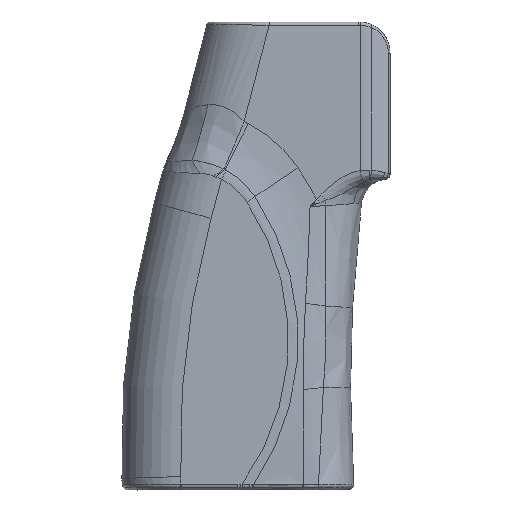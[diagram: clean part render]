
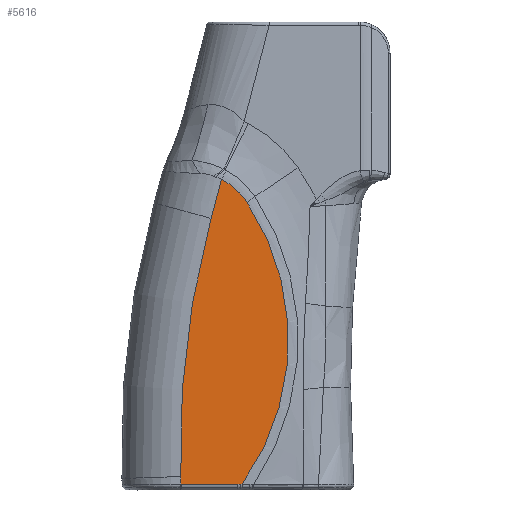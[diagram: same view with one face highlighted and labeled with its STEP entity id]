
A CAD part, left-side view. The second image highlights one B-rep face of the part: STEP entity #5616.
In plain terms, the highlighted planar face has unit normal (-1, 0, 0).
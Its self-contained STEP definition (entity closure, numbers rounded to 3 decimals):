
#102=PLANE('',#6028);
#186=LINE('',#9908,#366);
#366=VECTOR('',#6651,10.);
#677=FACE_OUTER_BOUND('',#1051,.T.);
#1051=EDGE_LOOP('',(#4062,#4063,#4064,#4065,#4066,#4067,#4068,#4069,#4070,
#4071));
#1429=CIRCLE('',#6029,50.737);
#1430=CIRCLE('',#6030,13.96);
#1431=CIRCLE('',#6031,1010.767);
#1432=CIRCLE('',#6032,178.004);
#1433=CIRCLE('',#6033,103.75);
#1751=B_SPLINE_CURVE_WITH_KNOTS('',3,(#9899,#9900,#9901,#9902),
 .UNSPECIFIED.,.F.,.F.,(4,4),(0.,0.054),.UNSPECIFIED.);
#1753=B_SPLINE_CURVE_WITH_KNOTS('',3,(#9932,#9933,#9934,#9935),
 .UNSPECIFIED.,.F.,.F.,(4,4),(0.,0.001),.UNSPECIFIED.);
#1755=B_SPLINE_CURVE_WITH_KNOTS('',3,(#9956,#9957,#9958,#9959),
 .UNSPECIFIED.,.F.,.F.,(4,4),(0.,0.033),
 .UNSPECIFIED.);
#1761=B_SPLINE_CURVE_WITH_KNOTS('',3,(#10067,#10068,#10069,#10070),
 .UNSPECIFIED.,.F.,.F.,(4,4),(0.,0.001),
 .UNSPECIFIED.);
#2205=VERTEX_POINT('',#9838);
#2207=VERTEX_POINT('',#9889);
#2210=VERTEX_POINT('',#9897);
#2211=VERTEX_POINT('',#9904);
#2213=VERTEX_POINT('',#9925);
#2218=VERTEX_POINT('',#9994);
#2275=VERTEX_POINT('',#10916);
#2276=VERTEX_POINT('',#10918);
#2277=VERTEX_POINT('',#10920);
#2278=VERTEX_POINT('',#10922);
#2842=EDGE_CURVE('',#2210,#2207,#1751,.T.);
#2845=EDGE_CURVE('',#2207,#2211,#186,.T.);
#2848=EDGE_CURVE('',#2211,#2213,#1753,.T.);
#2850=EDGE_CURVE('',#2205,#2210,#1755,.T.);
#2862=EDGE_CURVE('',#2213,#2218,#1761,.T.);
#2949=EDGE_CURVE('',#2275,#2205,#1429,.T.);
#2950=EDGE_CURVE('',#2276,#2275,#1430,.T.);
#2951=EDGE_CURVE('',#2277,#2276,#1431,.T.);
#2952=EDGE_CURVE('',#2278,#2277,#1432,.T.);
#2953=EDGE_CURVE('',#2218,#2278,#1433,.T.);
#4062=ORIENTED_EDGE('',*,*,#2862,.F.);
#4063=ORIENTED_EDGE('',*,*,#2848,.F.);
#4064=ORIENTED_EDGE('',*,*,#2845,.F.);
#4065=ORIENTED_EDGE('',*,*,#2842,.F.);
#4066=ORIENTED_EDGE('',*,*,#2850,.F.);
#4067=ORIENTED_EDGE('',*,*,#2949,.F.);
#4068=ORIENTED_EDGE('',*,*,#2950,.F.);
#4069=ORIENTED_EDGE('',*,*,#2951,.F.);
#4070=ORIENTED_EDGE('',*,*,#2952,.F.);
#4071=ORIENTED_EDGE('',*,*,#2953,.F.);
#5616=ADVANCED_FACE('',(#677),#102,.T.);
#6028=AXIS2_PLACEMENT_3D('',#10915,#6732,#6733);
#6029=AXIS2_PLACEMENT_3D('',#10917,#6734,#6735);
#6030=AXIS2_PLACEMENT_3D('',#10919,#6736,#6737);
#6031=AXIS2_PLACEMENT_3D('',#10921,#6738,#6739);
#6032=AXIS2_PLACEMENT_3D('',#10923,#6740,#6741);
#6033=AXIS2_PLACEMENT_3D('',#10924,#6742,#6743);
#6651=DIRECTION('',(0.,1.,0.));
#6732=DIRECTION('center_axis',(-1.,0.,0.));
#6733=DIRECTION('ref_axis',(0.,-1.,0.));
#6734=DIRECTION('center_axis',(1.,0.,0.));
#6735=DIRECTION('ref_axis',(0.,-0.988,-0.153));
#6736=DIRECTION('center_axis',(1.,0.,0.));
#6737=DIRECTION('ref_axis',(0.,-0.663,0.748));
#6738=DIRECTION('center_axis',(-1.,0.,0.));
#6739=DIRECTION('ref_axis',(0.,-0.966,-0.259));
#6740=DIRECTION('center_axis',(1.,0.,0.));
#6741=DIRECTION('ref_axis',(0.,0.993,0.116));
#6742=DIRECTION('center_axis',(-1.,0.,0.));
#6743=DIRECTION('ref_axis',(0.,-0.999,-0.051));
#9838=CARTESIAN_POINT('',(11.668,-119.652,-65.824));
#9889=CARTESIAN_POINT('',(11.668,-118.787,-65.836));
#9897=CARTESIAN_POINT('',(11.668,-119.325,-65.832));
#9899=CARTESIAN_POINT('Ctrl Pts',(11.668,-119.325,-65.832));
#9900=CARTESIAN_POINT('Ctrl Pts',(11.668,-119.146,-65.835));
#9901=CARTESIAN_POINT('Ctrl Pts',(11.668,-118.967,-65.836));
#9902=CARTESIAN_POINT('Ctrl Pts',(11.668,-118.787,-65.836));
#9904=CARTESIAN_POINT('',(11.668,-107.204,-65.836));
#9908=CARTESIAN_POINT('',(11.668,-119.773,-65.836));
#9925=CARTESIAN_POINT('',(11.668,-107.197,-65.836));
#9932=CARTESIAN_POINT('Ctrl Pts',(11.668,-107.204,-65.836));
#9933=CARTESIAN_POINT('Ctrl Pts',(11.668,-107.202,-65.836));
#9934=CARTESIAN_POINT('Ctrl Pts',(11.668,-107.199,-65.836));
#9935=CARTESIAN_POINT('Ctrl Pts',(11.668,-107.197,-65.836));
#9956=CARTESIAN_POINT('Ctrl Pts',(11.668,-119.652,-65.824));
#9957=CARTESIAN_POINT('Ctrl Pts',(11.668,-119.543,-65.828));
#9958=CARTESIAN_POINT('Ctrl Pts',(11.668,-119.434,-65.831));
#9959=CARTESIAN_POINT('Ctrl Pts',(11.668,-119.325,-65.832));
#9994=CARTESIAN_POINT('',(11.668,-107.19,-65.836));
#10067=CARTESIAN_POINT('Ctrl Pts',(11.668,-107.197,-65.836));
#10068=CARTESIAN_POINT('Ctrl Pts',(11.668,-107.195,-65.836));
#10069=CARTESIAN_POINT('Ctrl Pts',(11.668,-107.193,-65.836));
#10070=CARTESIAN_POINT('Ctrl Pts',(11.668,-107.19,-65.836));
#10915=CARTESIAN_POINT('Origin',(11.668,-118.964,-29.797));
#10916=CARTESIAN_POINT('',(11.668,-120.61,-8.274));
#10917=CARTESIAN_POINT('Origin',(11.668,-78.351,-36.354));
#10918=CARTESIAN_POINT('',(11.668,-115.458,-3.633));
#10919=CARTESIAN_POINT('Origin',(11.668,-108.983,-16.));
#10920=CARTESIAN_POINT('',(11.668,-113.317,-11.621));
#10921=CARTESIAN_POINT('Origin',(11.668,861.892,254.118));
#10922=CARTESIAN_POINT('',(11.668,-107.15,-64.253));
#10923=CARTESIAN_POINT('Origin',(11.668,-285.059,-58.42));
#10924=CARTESIAN_POINT('Origin',(11.668,-3.456,-67.652));
